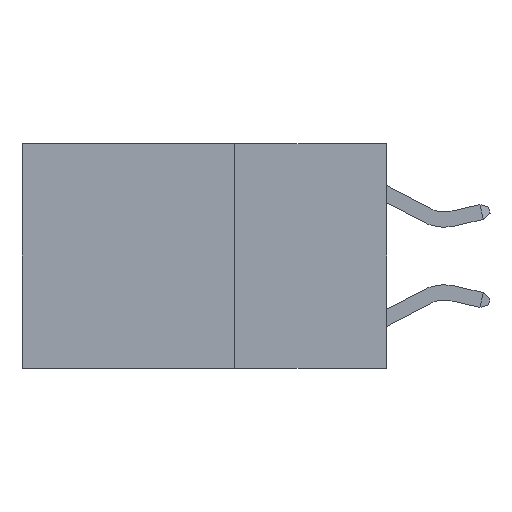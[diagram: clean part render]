
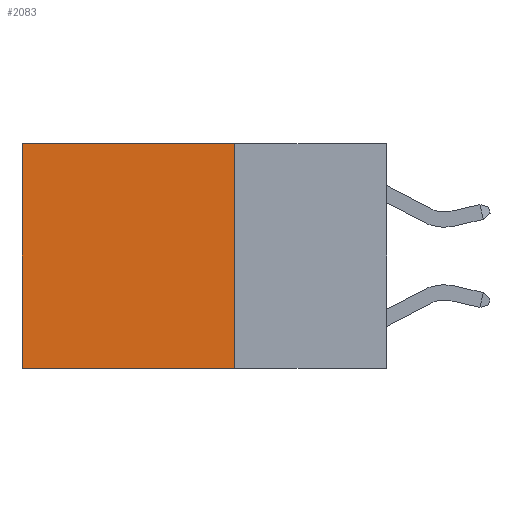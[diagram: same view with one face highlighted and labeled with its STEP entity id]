
A CAD part, left-side view. The second image highlights one B-rep face of the part: STEP entity #2083.
In plain terms, the highlighted planar face has unit normal (-1, 0, 0).
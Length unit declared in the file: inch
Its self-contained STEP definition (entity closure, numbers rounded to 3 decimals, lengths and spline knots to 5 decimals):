
#430 = EDGE_CURVE ( 'NONE', #1804, #13639, #2313, .T. ) ;
#628 = DIRECTION ( 'NONE',  ( 0., 0., -1. ) ) ;
#1804 = VERTEX_POINT ( 'NONE', #14013 ) ;
#1847 = EDGE_CURVE ( 'NONE', #13639, #13286, #19109, .T. ) ;
#2083 = ADVANCED_FACE ( 'NONE', ( #19288 ), #5698, .F. ) ;
#2134 = VECTOR ( 'NONE', #19265, 39.37008 ) ;
#2199 = CARTESIAN_POINT ( 'NONE',  ( 0.2625, 0.25, 0. ) ) ;
#2313 = LINE ( 'NONE', #2199, #21528 ) ;
#2693 = CARTESIAN_POINT ( 'NONE',  ( 0.2625, 0.25, 0. ) ) ;
#3460 = LINE ( 'NONE', #20155, #11111 ) ;
#3959 = CARTESIAN_POINT ( 'NONE',  ( 0.2625, 0.25, -0.37 ) ) ;
#5003 = DIRECTION ( 'NONE',  ( 0., 0., -1. ) ) ;
#5698 = PLANE ( 'NONE',  #18654 ) ;
#5731 = DIRECTION ( 'NONE',  ( 0., 1., 0. ) ) ;
#5919 = EDGE_LOOP ( 'NONE', ( #13324, #10092, #20074, #19612 ) ) ;
#6027 = EDGE_CURVE ( 'NONE', #10815, #13286, #3460, .T. ) ;
#7357 = CARTESIAN_POINT ( 'NONE',  ( 0.2625, 0.25, 0. ) ) ;
#10092 = ORIENTED_EDGE ( 'NONE', *, *, #1847, .F. ) ;
#10815 = VERTEX_POINT ( 'NONE', #17125 ) ;
#11111 = VECTOR ( 'NONE', #5003, 39.37008 ) ;
#11882 = VECTOR ( 'NONE', #5731, 39.37008 ) ;
#13286 = VERTEX_POINT ( 'NONE', #14609 ) ;
#13324 = ORIENTED_EDGE ( 'NONE', *, *, #6027, .T. ) ;
#13639 = VERTEX_POINT ( 'NONE', #14247 ) ;
#14013 = CARTESIAN_POINT ( 'NONE',  ( 0.2625, 0.25, 0. ) ) ;
#14084 = DIRECTION ( 'NONE',  ( 0., 0., -1. ) ) ;
#14247 = CARTESIAN_POINT ( 'NONE',  ( 0.2625, 0.25, -0.37 ) ) ;
#14609 = CARTESIAN_POINT ( 'NONE',  ( 0.2625, 0.6, -0.37 ) ) ;
#17125 = CARTESIAN_POINT ( 'NONE',  ( 0.2625, 0.6, 0. ) ) ;
#17800 = EDGE_CURVE ( 'NONE', #1804, #10815, #19606, .T. ) ;
#18654 = AXIS2_PLACEMENT_3D ( 'NONE', #7357, #18958, #14084 ) ;
#18958 = DIRECTION ( 'NONE',  ( 1., 0., 0. ) ) ;
#19109 = LINE ( 'NONE', #3959, #11882 ) ;
#19265 = DIRECTION ( 'NONE',  ( 0., 1., 0. ) ) ;
#19288 = FACE_OUTER_BOUND ( 'NONE', #5919, .T. ) ;
#19606 = LINE ( 'NONE', #2693, #2134 ) ;
#19612 = ORIENTED_EDGE ( 'NONE', *, *, #17800, .T. ) ;
#20074 = ORIENTED_EDGE ( 'NONE', *, *, #430, .F. ) ;
#20155 = CARTESIAN_POINT ( 'NONE',  ( 0.2625, 0.6, 0. ) ) ;
#21528 = VECTOR ( 'NONE', #628, 39.37008 ) ;
